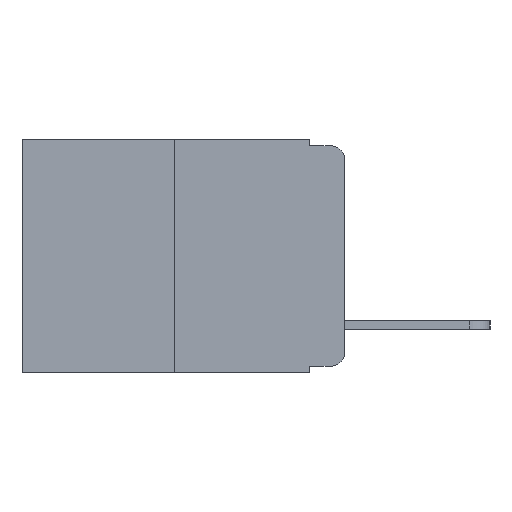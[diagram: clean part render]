
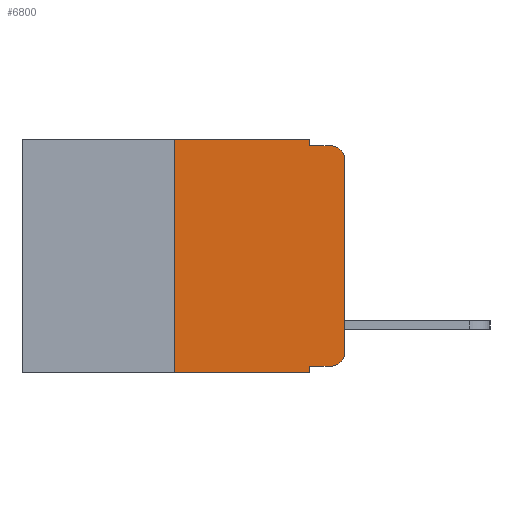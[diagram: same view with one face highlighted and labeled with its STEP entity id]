
A CAD part, left-side view. The second image highlights one B-rep face of the part: STEP entity #6800.
In plain terms, the highlighted planar face has unit normal (-1, 0, 0).
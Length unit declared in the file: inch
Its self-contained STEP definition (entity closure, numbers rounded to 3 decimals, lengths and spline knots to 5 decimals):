
#15 = CIRCLE ( 'NONE', #10620, 0.02 ) ;
#107 = CARTESIAN_POINT ( 'NONE',  ( 0., 0.051, 0. ) ) ;
#307 = DIRECTION ( 'NONE',  ( 0., -1., 0. ) ) ;
#551 = ORIENTED_EDGE ( 'NONE', *, *, #13489, .T. ) ;
#582 = ORIENTED_EDGE ( 'NONE', *, *, #13521, .T. ) ;
#673 = ORIENTED_EDGE ( 'NONE', *, *, #13524, .F. ) ;
#695 = VERTEX_POINT ( 'NONE', #5952 ) ;
#809 = ORIENTED_EDGE ( 'NONE', *, *, #13541, .F. ) ;
#870 = CARTESIAN_POINT ( 'NONE',  ( 0., 0.02, -0.313 ) ) ;
#902 = ORIENTED_EDGE ( 'NONE', *, *, #7592, .F. ) ;
#928 = ORIENTED_EDGE ( 'NONE', *, *, #13555, .F. ) ;
#936 = DIRECTION ( 'NONE',  ( -1., 0., 0. ) ) ;
#944 = CARTESIAN_POINT ( 'NONE',  ( 0., 0.051, -0.01 ) ) ;
#974 = DIRECTION ( 'NONE',  ( 0., 0., 1. ) ) ;
#1003 = VERTEX_POINT ( 'NONE', #8174 ) ;
#1062 = ORIENTED_EDGE ( 'NONE', *, *, #12543, .T. ) ;
#1097 = DIRECTION ( 'NONE',  ( 0., 0., -1. ) ) ;
#1109 = DIRECTION ( 'NONE',  ( 0., -1., 0. ) ) ;
#1135 = CARTESIAN_POINT ( 'NONE',  ( 0., 0.473, -0.343 ) ) ;
#1178 = ORIENTED_EDGE ( 'NONE', *, *, #13574, .F. ) ;
#1194 = VERTEX_POINT ( 'NONE', #12839 ) ;
#1256 = ORIENTED_EDGE ( 'NONE', *, *, #13588, .T. ) ;
#1337 = DIRECTION ( 'NONE',  ( 0., 0., -1. ) ) ;
#1407 = DIRECTION ( 'NONE',  ( -1., 0., 0. ) ) ;
#1411 = ORIENTED_EDGE ( 'NONE', *, *, #13592, .T. ) ;
#1436 = VERTEX_POINT ( 'NONE', #4236 ) ;
#1927 = DIRECTION ( 'NONE',  ( 0., 0., 1. ) ) ;
#1954 = CARTESIAN_POINT ( 'NONE',  ( 0., 0.051, -0.333 ) ) ;
#1985 = CARTESIAN_POINT ( 'NONE',  ( 0., 0.25, 0. ) ) ;
#2016 = LINE ( 'NONE', #1954, #12644 ) ;
#2223 = CARTESIAN_POINT ( 'NONE',  ( 0., 0., -0.03 ) ) ;
#2426 = VECTOR ( 'NONE', #1927, 39.37008 ) ;
#2984 = CARTESIAN_POINT ( 'NONE',  ( 0., 0.051, -0.343 ) ) ;
#3138 = VECTOR ( 'NONE', #7180, 39.37008 ) ;
#3729 = DIRECTION ( 'NONE',  ( 0., -1., 0. ) ) ;
#3745 = CARTESIAN_POINT ( 'NONE',  ( 0., 0.473, 0. ) ) ;
#4074 = VECTOR ( 'NONE', #1109, 39.37008 ) ;
#4236 = CARTESIAN_POINT ( 'NONE',  ( 0., 0.051, 0. ) ) ;
#4298 = LINE ( 'NONE', #6437, #6552 ) ;
#5214 = CIRCLE ( 'NONE', #11916, 0.02 ) ;
#5568 = VERTEX_POINT ( 'NONE', #6830 ) ;
#5616 = LINE ( 'NONE', #3745, #10581 ) ;
#5849 = CARTESIAN_POINT ( 'NONE',  ( 0., 0.02, -0.01 ) ) ;
#5881 = VECTOR ( 'NONE', #13596, 39.37008 ) ;
#5952 = CARTESIAN_POINT ( 'NONE',  ( 0., 0.051, -0.333 ) ) ;
#6437 = CARTESIAN_POINT ( 'NONE',  ( 0., 0., 0. ) ) ;
#6552 = VECTOR ( 'NONE', #974, 39.37008 ) ;
#6553 = CARTESIAN_POINT ( 'NONE',  ( 0., 0.02, -0.03 ) ) ;
#6800 = ADVANCED_FACE ( 'NONE', ( #9086 ), #12629, .F. ) ;
#6830 = CARTESIAN_POINT ( 'NONE',  ( 0., 0.25, 0. ) ) ;
#7025 = CARTESIAN_POINT ( 'NONE',  ( 0., 0.051, -0.01 ) ) ;
#7180 = DIRECTION ( 'NONE',  ( 0., -1., 0. ) ) ;
#7192 = AXIS2_PLACEMENT_3D ( 'NONE', #12774, #12568, #12554 ) ;
#7592 = EDGE_CURVE ( 'NONE', #5568, #1436, #5616, .T. ) ;
#7959 = VECTOR ( 'NONE', #1097, 39.37008 ) ;
#8174 = CARTESIAN_POINT ( 'NONE',  ( 0., 0.02, -0.333 ) ) ;
#8271 = EDGE_LOOP ( 'NONE', ( #551, #582, #673, #809, #902, #928, #1062, #1178, #1256, #1411 ) ) ;
#8510 = VERTEX_POINT ( 'NONE', #2223 ) ;
#8559 = LINE ( 'NONE', #107, #7959 ) ;
#9086 = FACE_OUTER_BOUND ( 'NONE', #8271, .T. ) ;
#9095 = VERTEX_POINT ( 'NONE', #5849 ) ;
#9169 = LINE ( 'NONE', #7025, #3138 ) ;
#9859 = CARTESIAN_POINT ( 'NONE',  ( 0., 0.25, -0.343 ) ) ;
#10485 = VERTEX_POINT ( 'NONE', #944 ) ;
#10581 = VECTOR ( 'NONE', #3729, 39.37008 ) ;
#10620 = AXIS2_PLACEMENT_3D ( 'NONE', #6553, #936, #13670 ) ;
#10822 = LINE ( 'NONE', #1985, #2426 ) ;
#11153 = VERTEX_POINT ( 'NONE', #9859 ) ;
#11916 = AXIS2_PLACEMENT_3D ( 'NONE', #870, #1407, #1337 ) ;
#12109 = LINE ( 'NONE', #1135, #4074 ) ;
#12362 = VERTEX_POINT ( 'NONE', #2984 ) ;
#12543 = EDGE_CURVE ( 'NONE', #11153, #12362, #12109, .T. ) ;
#12554 = DIRECTION ( 'NONE',  ( 0., 0., -1. ) ) ;
#12568 = DIRECTION ( 'NONE',  ( 1., 0., 0. ) ) ;
#12629 = PLANE ( 'NONE',  #7192 ) ;
#12644 = VECTOR ( 'NONE', #307, 39.37008 ) ;
#12774 = CARTESIAN_POINT ( 'NONE',  ( 0., 0.473, 0. ) ) ;
#12839 = CARTESIAN_POINT ( 'NONE',  ( 0., 0., -0.313 ) ) ;
#13489 = EDGE_CURVE ( 'NONE', #1194, #8510, #4298, .T. ) ;
#13509 = LINE ( 'NONE', #13621, #5881 ) ;
#13521 = EDGE_CURVE ( 'NONE', #8510, #9095, #15, .T. ) ;
#13524 = EDGE_CURVE ( 'NONE', #10485, #9095, #9169, .T. ) ;
#13541 = EDGE_CURVE ( 'NONE', #1436, #10485, #13509, .T. ) ;
#13555 = EDGE_CURVE ( 'NONE', #11153, #5568, #10822, .T. ) ;
#13574 = EDGE_CURVE ( 'NONE', #695, #12362, #8559, .T. ) ;
#13588 = EDGE_CURVE ( 'NONE', #695, #1003, #2016, .T. ) ;
#13592 = EDGE_CURVE ( 'NONE', #1003, #1194, #5214, .T. ) ;
#13596 = DIRECTION ( 'NONE',  ( 0., 0., -1. ) ) ;
#13621 = CARTESIAN_POINT ( 'NONE',  ( 0., 0.051, 0. ) ) ;
#13670 = DIRECTION ( 'NONE',  ( 0., 0., -1. ) ) ;
